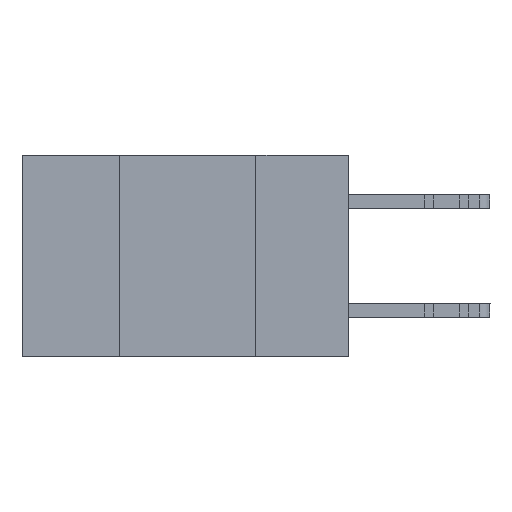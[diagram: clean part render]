
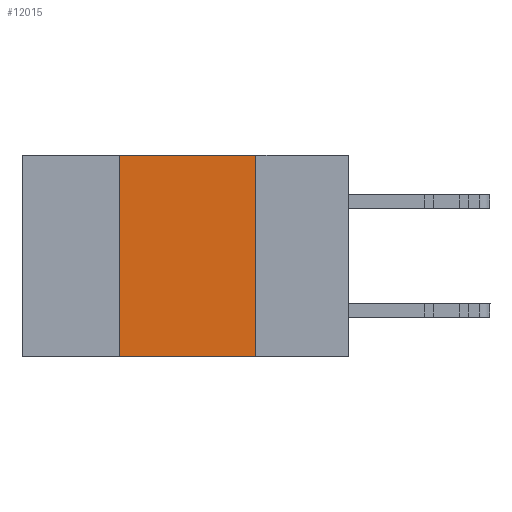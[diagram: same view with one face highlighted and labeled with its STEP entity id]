
A CAD part, left-side view. The second image highlights one B-rep face of the part: STEP entity #12015.
In plain terms, the highlighted planar face has unit normal (-1, 0, 0).
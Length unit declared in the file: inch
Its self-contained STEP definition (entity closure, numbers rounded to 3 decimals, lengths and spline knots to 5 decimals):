
#174 = CARTESIAN_POINT ( 'NONE',  ( 0., 0.42, 0. ) ) ;
#454 = VECTOR ( 'NONE', #10738, 39.37008 ) ;
#2633 = VECTOR ( 'NONE', #7201, 39.37008 ) ;
#6398 = PLANE ( 'NONE',  #25453 ) ;
#7201 = DIRECTION ( 'NONE',  ( 0., 0., 1. ) ) ;
#7239 = CARTESIAN_POINT ( 'NONE',  ( 0., 0.6, -0.37 ) ) ;
#7310 = VECTOR ( 'NONE', #10100, 39.37008 ) ;
#7647 = CARTESIAN_POINT ( 'NONE',  ( 0., 0.17, -0.37 ) ) ;
#8372 = CARTESIAN_POINT ( 'NONE',  ( 0., 0.17, 0. ) ) ;
#9270 = CARTESIAN_POINT ( 'NONE',  ( 0., 0.42, 0. ) ) ;
#9905 = CARTESIAN_POINT ( 'NONE',  ( 0., 0.6, 0. ) ) ;
#10100 = DIRECTION ( 'NONE',  ( 0., -1., 0. ) ) ;
#10327 = ORIENTED_EDGE ( 'NONE', *, *, #21365, .F. ) ;
#10738 = DIRECTION ( 'NONE',  ( 0., 0., -1. ) ) ;
#11123 = DIRECTION ( 'NONE',  ( 0., 0., -1. ) ) ;
#11579 = VECTOR ( 'NONE', #27753, 39.37008 ) ;
#12015 = ADVANCED_FACE ( 'NONE', ( #22905 ), #6398, .F. ) ;
#12960 = LINE ( 'NONE', #9905, #7310 ) ;
#13654 = VERTEX_POINT ( 'NONE', #25379 ) ;
#14408 = EDGE_CURVE ( 'NONE', #23203, #13654, #12960, .T. ) ;
#15159 = LINE ( 'NONE', #7239, #11579 ) ;
#15793 = CARTESIAN_POINT ( 'NONE',  ( 0., 0.42, -0.37 ) ) ;
#16935 = ORIENTED_EDGE ( 'NONE', *, *, #28919, .T. ) ;
#20102 = DIRECTION ( 'NONE',  ( 1., 0., 0. ) ) ;
#21365 = EDGE_CURVE ( 'NONE', #27560, #23203, #24946, .T. ) ;
#22453 = CARTESIAN_POINT ( 'NONE',  ( 0., 0.6, 0. ) ) ;
#22554 = EDGE_CURVE ( 'NONE', #13654, #23966, #24524, .T. ) ;
#22905 = FACE_OUTER_BOUND ( 'NONE', #25510, .T. ) ;
#23203 = VERTEX_POINT ( 'NONE', #174 ) ;
#23966 = VERTEX_POINT ( 'NONE', #7647 ) ;
#24239 = ORIENTED_EDGE ( 'NONE', *, *, #14408, .F. ) ;
#24524 = LINE ( 'NONE', #8372, #454 ) ;
#24946 = LINE ( 'NONE', #9270, #2633 ) ;
#25379 = CARTESIAN_POINT ( 'NONE',  ( 0., 0.17, 0. ) ) ;
#25453 = AXIS2_PLACEMENT_3D ( 'NONE', #22453, #20102, #11123 ) ;
#25510 = EDGE_LOOP ( 'NONE', ( #26857, #24239, #10327, #16935 ) ) ;
#26857 = ORIENTED_EDGE ( 'NONE', *, *, #22554, .F. ) ;
#27560 = VERTEX_POINT ( 'NONE', #15793 ) ;
#27753 = DIRECTION ( 'NONE',  ( 0., -1., 0. ) ) ;
#28919 = EDGE_CURVE ( 'NONE', #27560, #23966, #15159, .T. ) ;
